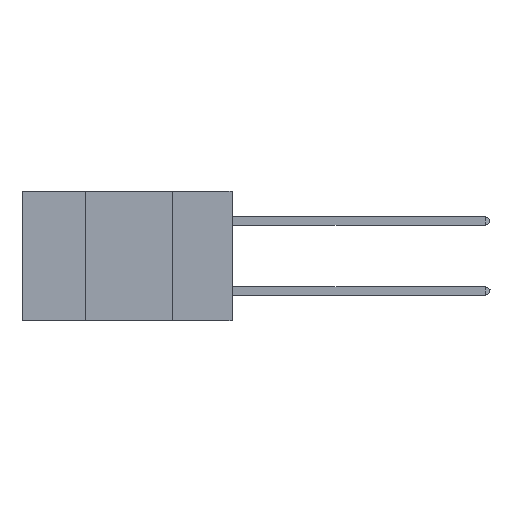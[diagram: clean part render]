
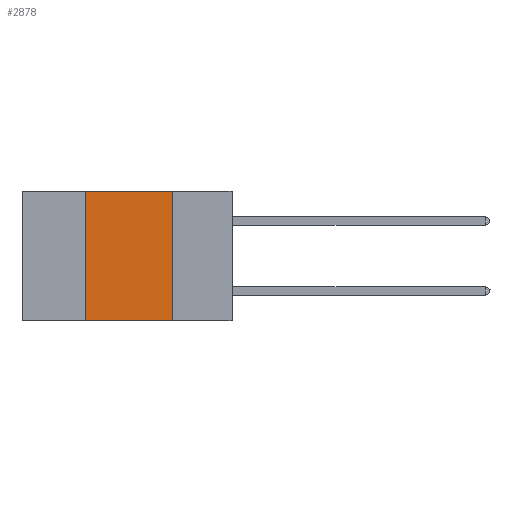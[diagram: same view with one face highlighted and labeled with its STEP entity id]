
A CAD part, left-side view. The second image highlights one B-rep face of the part: STEP entity #2878.
In plain terms, the highlighted planar face has unit normal (-1, 0, 0).
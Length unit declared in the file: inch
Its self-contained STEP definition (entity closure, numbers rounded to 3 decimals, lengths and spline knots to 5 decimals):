
#73 = DIRECTION ( 'NONE',  ( 0., -1., 0. ) ) ;
#81 = CARTESIAN_POINT ( 'NONE',  ( 0., 0.17, 0. ) ) ;
#644 = EDGE_CURVE ( 'NONE', #9461, #14879, #4201, .T. ) ;
#676 = DIRECTION ( 'NONE',  ( 0., 0., 1. ) ) ;
#1313 = LINE ( 'NONE', #12069, #2253 ) ;
#1539 = DIRECTION ( 'NONE',  ( 0., 0., -1. ) ) ;
#1913 = CARTESIAN_POINT ( 'NONE',  ( 0., 0.42, 0. ) ) ;
#2230 = CARTESIAN_POINT ( 'NONE',  ( 0., 0.17, -0.37 ) ) ;
#2253 = VECTOR ( 'NONE', #18067, 39.37008 ) ;
#2623 = DIRECTION ( 'NONE',  ( 0., 0., -1. ) ) ;
#2878 = ADVANCED_FACE ( 'NONE', ( #16149 ), #18494, .F. ) ;
#3450 = CARTESIAN_POINT ( 'NONE',  ( 0., 0.42, 0. ) ) ;
#4201 = LINE ( 'NONE', #11303, #18341 ) ;
#4447 = CARTESIAN_POINT ( 'NONE',  ( 0., 0.17, 0. ) ) ;
#5177 = EDGE_LOOP ( 'NONE', ( #11386, #15079, #17867, #12978 ) ) ;
#5542 = VECTOR ( 'NONE', #1539, 39.37008 ) ;
#6994 = EDGE_CURVE ( 'NONE', #13622, #15265, #1313, .T. ) ;
#7226 = VECTOR ( 'NONE', #676, 39.37008 ) ;
#8359 = LINE ( 'NONE', #3450, #7226 ) ;
#8451 = EDGE_CURVE ( 'NONE', #15265, #14879, #9391, .T. ) ;
#8665 = CARTESIAN_POINT ( 'NONE',  ( 0., 0.42, -0.37 ) ) ;
#9391 = LINE ( 'NONE', #81, #5542 ) ;
#9461 = VERTEX_POINT ( 'NONE', #8665 ) ;
#11303 = CARTESIAN_POINT ( 'NONE',  ( 0., 0.6, -0.37 ) ) ;
#11386 = ORIENTED_EDGE ( 'NONE', *, *, #8451, .F. ) ;
#11447 = EDGE_CURVE ( 'NONE', #9461, #13622, #8359, .T. ) ;
#12069 = CARTESIAN_POINT ( 'NONE',  ( 0., 0.6, 0. ) ) ;
#12978 = ORIENTED_EDGE ( 'NONE', *, *, #644, .T. ) ;
#13325 = AXIS2_PLACEMENT_3D ( 'NONE', #17033, #15545, #2623 ) ;
#13622 = VERTEX_POINT ( 'NONE', #1913 ) ;
#14879 = VERTEX_POINT ( 'NONE', #2230 ) ;
#15079 = ORIENTED_EDGE ( 'NONE', *, *, #6994, .F. ) ;
#15265 = VERTEX_POINT ( 'NONE', #4447 ) ;
#15545 = DIRECTION ( 'NONE',  ( 1., 0., 0. ) ) ;
#16149 = FACE_OUTER_BOUND ( 'NONE', #5177, .T. ) ;
#17033 = CARTESIAN_POINT ( 'NONE',  ( 0., 0.6, 0. ) ) ;
#17867 = ORIENTED_EDGE ( 'NONE', *, *, #11447, .F. ) ;
#18067 = DIRECTION ( 'NONE',  ( 0., -1., 0. ) ) ;
#18341 = VECTOR ( 'NONE', #73, 39.37008 ) ;
#18494 = PLANE ( 'NONE',  #13325 ) ;
